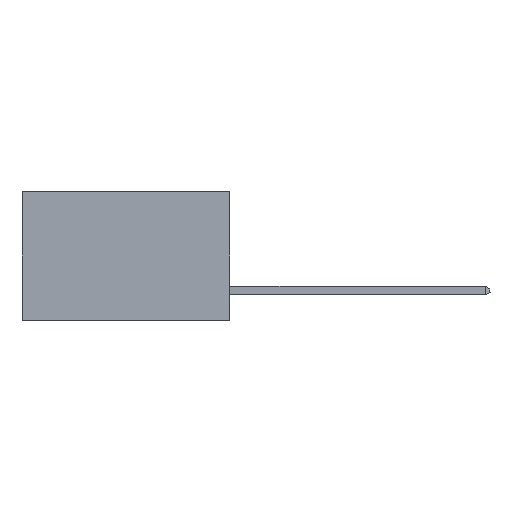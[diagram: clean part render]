
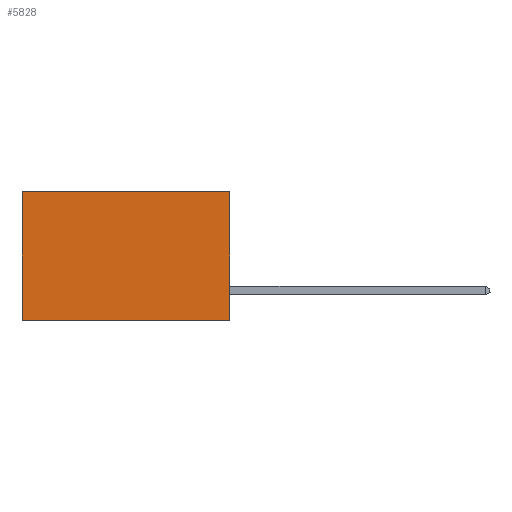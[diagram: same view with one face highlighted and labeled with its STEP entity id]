
A CAD part, left-side view. The second image highlights one B-rep face of the part: STEP entity #5828.
In plain terms, the highlighted planar face has unit normal (-1, 0, 0).
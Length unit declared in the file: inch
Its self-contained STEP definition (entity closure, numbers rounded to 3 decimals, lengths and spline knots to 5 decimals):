
#424 = VECTOR ( 'NONE', #15297, 39.37008 ) ;
#505 = AXIS2_PLACEMENT_3D ( 'NONE', #13071, #4380, #22060 ) ;
#658 = VECTOR ( 'NONE', #3146, 39.37008 ) ;
#738 = EDGE_CURVE ( 'NONE', #22002, #1778, #18629, .T. ) ;
#1778 = VERTEX_POINT ( 'NONE', #7573 ) ;
#1842 = VERTEX_POINT ( 'NONE', #13130 ) ;
#2012 = DIRECTION ( 'NONE',  ( 0., 1., 0. ) ) ;
#2289 = CARTESIAN_POINT ( 'NONE',  ( 0.298, 0., 0. ) ) ;
#2324 = PLANE ( 'NONE',  #505 ) ;
#2972 = VECTOR ( 'NONE', #14987, 39.37008 ) ;
#3146 = DIRECTION ( 'NONE',  ( 0., 1., 0. ) ) ;
#4380 = DIRECTION ( 'NONE',  ( 1., 0., 0. ) ) ;
#4526 = CARTESIAN_POINT ( 'NONE',  ( 0.298, 0., 0. ) ) ;
#4721 = CARTESIAN_POINT ( 'NONE',  ( 0.298, 0.6, -0.37 ) ) ;
#5285 = LINE ( 'NONE', #13831, #658 ) ;
#5828 = ADVANCED_FACE ( 'NONE', ( #22221 ), #2324, .F. ) ;
#6133 = ORIENTED_EDGE ( 'NONE', *, *, #738, .F. ) ;
#7173 = EDGE_LOOP ( 'NONE', ( #16476, #7276, #6133, #19723 ) ) ;
#7255 = EDGE_CURVE ( 'NONE', #1842, #16227, #13321, .T. ) ;
#7276 = ORIENTED_EDGE ( 'NONE', *, *, #14493, .F. ) ;
#7573 = CARTESIAN_POINT ( 'NONE',  ( 0.298, 0., -0.37 ) ) ;
#7577 = CARTESIAN_POINT ( 'NONE',  ( 0.298, 0., 0. ) ) ;
#10477 = LINE ( 'NONE', #7577, #14617 ) ;
#12978 = EDGE_CURVE ( 'NONE', #22002, #1842, #10477, .T. ) ;
#13071 = CARTESIAN_POINT ( 'NONE',  ( 0.298, 0., 0. ) ) ;
#13130 = CARTESIAN_POINT ( 'NONE',  ( 0.298, 0.6, 0. ) ) ;
#13321 = LINE ( 'NONE', #22294, #424 ) ;
#13831 = CARTESIAN_POINT ( 'NONE',  ( 0.298, 0., -0.37 ) ) ;
#14493 = EDGE_CURVE ( 'NONE', #1778, #16227, #5285, .T. ) ;
#14617 = VECTOR ( 'NONE', #2012, 39.37008 ) ;
#14987 = DIRECTION ( 'NONE',  ( 0., 0., -1. ) ) ;
#15297 = DIRECTION ( 'NONE',  ( 0., 0., -1. ) ) ;
#16227 = VERTEX_POINT ( 'NONE', #4721 ) ;
#16476 = ORIENTED_EDGE ( 'NONE', *, *, #7255, .T. ) ;
#18629 = LINE ( 'NONE', #4526, #2972 ) ;
#19723 = ORIENTED_EDGE ( 'NONE', *, *, #12978, .T. ) ;
#22002 = VERTEX_POINT ( 'NONE', #2289 ) ;
#22060 = DIRECTION ( 'NONE',  ( 0., 0., -1. ) ) ;
#22221 = FACE_OUTER_BOUND ( 'NONE', #7173, .T. ) ;
#22294 = CARTESIAN_POINT ( 'NONE',  ( 0.298, 0.6, 0. ) ) ;
